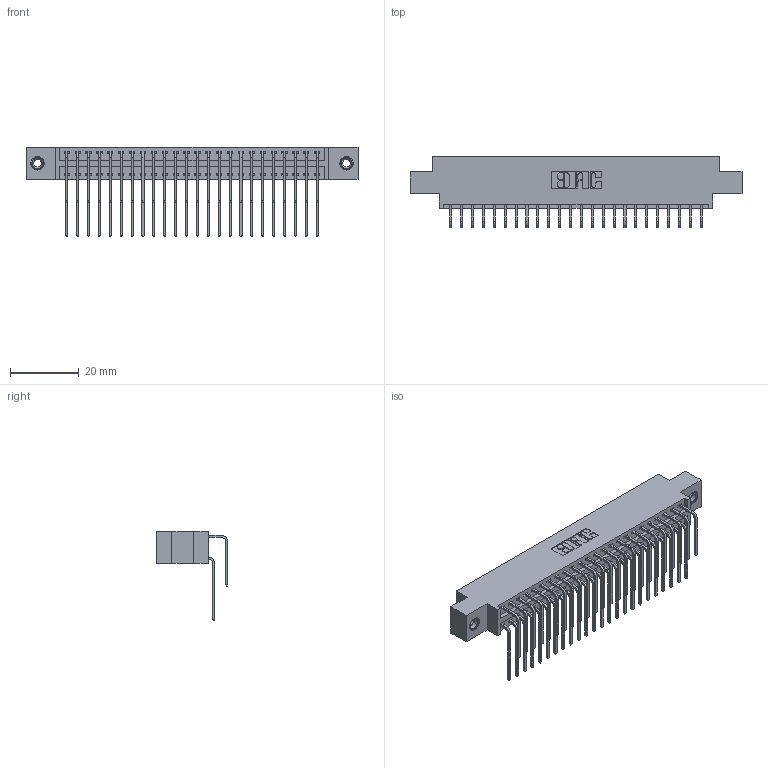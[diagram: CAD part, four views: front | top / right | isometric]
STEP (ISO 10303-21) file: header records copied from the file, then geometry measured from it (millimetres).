
FILE_DESCRIPTION (( 'STEP AP203' ), '1' );
FILE_NAME ('396-048-559-808.STEP', '2019-11-03T08:27:52', ( '' ), ( '' ), 'SwSTEP 2.0', 'SolidWorks 2016', '' );
FILE_SCHEMA (( 'CONFIG_CONTROL_DESIGN' ));
Length unit declared in the file: inch
Products named in the file (5): 345-292-001_559 Tail - 2; 345-250-001_345-250-003-102; 345-292-001_558 559 Tail - 1; 346 Part_0.170 Offset - 0.156 Dia-TI; 396-048-559-808
Assembly tree (51 placements, depth 2):
  396-048-559-808
    346 Part_0.170 Offset - 0.156 Dia-TI
    345-292-001_558 559 Tail - 1  x24
    345-292-001_559 Tail - 2  x24
    345-250-001_345-250-003-102  x2
Bounding box: 96.77 x 20.89 x 26.16 mm (x, y, z)
Volume: 9412.6 mm3; surface area: 14183.4 mm2
Topology: 51 solids, 51 shells, 2778 faces, 8205 edges, 5398 vertices
Faces by surface type: plane 1888, cylinder 874, cone 12, torus 4
Entity records: 21188 total; most frequent: CARTESIAN_POINT 3554, ORIENTED_EDGE 3430, DIRECTION 3181, EDGE_CURVE 1715, LINE 1427, VECTOR 1427, VERTEX_POINT 1136, AXIS2_PLACEMENT_3D 877
